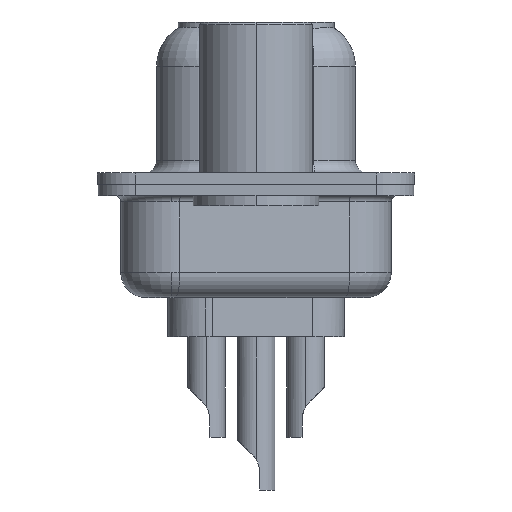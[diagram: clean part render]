
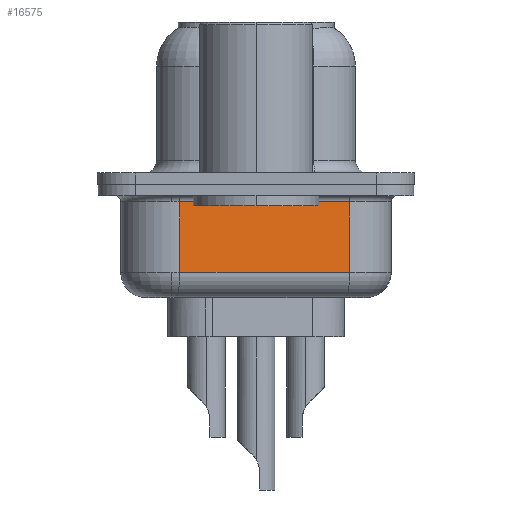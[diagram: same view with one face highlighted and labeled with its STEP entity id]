
A CAD part, left-side view. The second image highlights one B-rep face of the part: STEP entity #16575.
In plain terms, the highlighted planar face has unit normal (-0.985, -0.174, 0).
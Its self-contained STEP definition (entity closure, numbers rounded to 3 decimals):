
#687 = EDGE_CURVE ( 'NONE', #24780, #9002, #3857, .T. ) ;
#1123 = VERTEX_POINT ( 'NONE', #11932 ) ;
#1351 = DIRECTION ( 'NONE',  ( -0.174, 0.985, 0. ) ) ;
#3511 = EDGE_CURVE ( 'NONE', #9002, #4539, #18426, .T. ) ;
#3857 = LINE ( 'NONE', #10561, #13689 ) ;
#4539 = VERTEX_POINT ( 'NONE', #24239 ) ;
#4777 = EDGE_CURVE ( 'NONE', #1123, #24780, #7289, .T. ) ;
#5175 = DIRECTION ( 'NONE',  ( -0.174, 0.985, 0. ) ) ;
#5515 = CARTESIAN_POINT ( 'NONE',  ( 2.925, 3.028, -3.5 ) ) ;
#6695 = DIRECTION ( 'NONE',  ( 0., 0., 1. ) ) ;
#7289 = LINE ( 'NONE', #5515, #17752 ) ;
#7454 = DIRECTION ( 'NONE',  ( 0., 0., 1. ) ) ;
#8218 = CARTESIAN_POINT ( 'NONE',  ( 4.116, -3.722, -0.7 ) ) ;
#8590 = VECTOR ( 'NONE', #1351, 1000. ) ;
#9002 = VERTEX_POINT ( 'NONE', #8218 ) ;
#9094 = CARTESIAN_POINT ( 'NONE',  ( 4.116, -3.722, -3.5 ) ) ;
#10561 = CARTESIAN_POINT ( 'NONE',  ( 4.116, -3.722, -4.5 ) ) ;
#11932 = CARTESIAN_POINT ( 'NONE',  ( 2.925, 3.028, -3.5 ) ) ;
#13689 = VECTOR ( 'NONE', #6695, 1000. ) ;
#13857 = LINE ( 'NONE', #21092, #23698 ) ;
#16575 = ADVANCED_FACE ( 'NONE', ( #19688 ), #18843, .F. ) ;
#16767 = ORIENTED_EDGE ( 'NONE', *, *, #18751, .F. ) ;
#16947 = DIRECTION ( 'NONE',  ( 0.985, 0.174, 0. ) ) ;
#17099 = CARTESIAN_POINT ( 'NONE',  ( 2.925, 3.028, -0.7 ) ) ;
#17752 = VECTOR ( 'NONE', #19246, 1000. ) ;
#18426 = LINE ( 'NONE', #17099, #8590 ) ;
#18751 = EDGE_CURVE ( 'NONE', #1123, #4539, #13857, .T. ) ;
#18843 = PLANE ( 'NONE',  #24034 ) ;
#19246 = DIRECTION ( 'NONE',  ( 0.174, -0.985, 0. ) ) ;
#19281 = ORIENTED_EDGE ( 'NONE', *, *, #687, .T. ) ;
#19688 = FACE_OUTER_BOUND ( 'NONE', #22168, .T. ) ;
#21092 = CARTESIAN_POINT ( 'NONE',  ( 2.925, 3.028, -4.5 ) ) ;
#22168 = EDGE_LOOP ( 'NONE', ( #16767, #22489, #19281, #25109 ) ) ;
#22489 = ORIENTED_EDGE ( 'NONE', *, *, #4777, .T. ) ;
#23698 = VECTOR ( 'NONE', #7454, 1000. ) ;
#24034 = AXIS2_PLACEMENT_3D ( 'NONE', #24734, #16947, #5175 ) ;
#24239 = CARTESIAN_POINT ( 'NONE',  ( 2.925, 3.028, -0.7 ) ) ;
#24734 = CARTESIAN_POINT ( 'NONE',  ( 2.925, 3.028, -4.5 ) ) ;
#24780 = VERTEX_POINT ( 'NONE', #9094 ) ;
#25109 = ORIENTED_EDGE ( 'NONE', *, *, #3511, .T. ) ;
